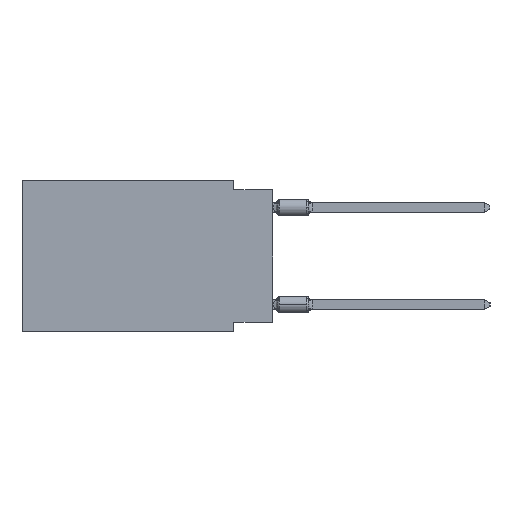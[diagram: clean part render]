
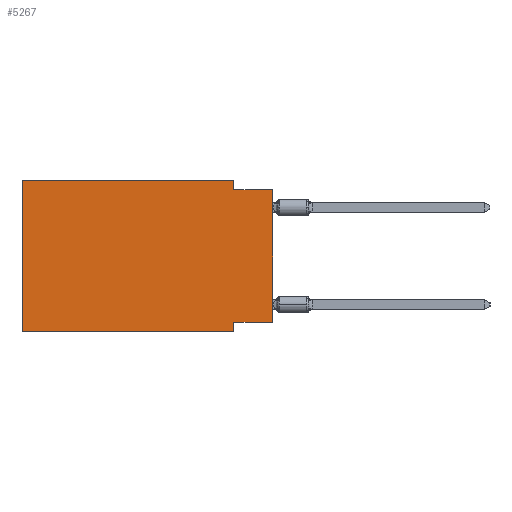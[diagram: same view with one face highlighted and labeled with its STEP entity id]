
A CAD part, left-side view. The second image highlights one B-rep face of the part: STEP entity #5267.
In plain terms, the highlighted planar face has unit normal (-1, 0, 0).
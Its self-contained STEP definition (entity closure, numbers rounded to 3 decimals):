
#580 = EDGE_CURVE ( 'NONE', #13527, #42944, #2707, .T. ) ;
#1333 = CARTESIAN_POINT ( 'NONE',  ( 0., 16.383, -9.906 ) ) ;
#2685 = EDGE_LOOP ( 'NONE', ( #35962, #48918, #42064, #32607, #46112, #20732, #15346, #41713 ) ) ;
#2707 = LINE ( 'NONE', #3240, #50632 ) ;
#3240 = CARTESIAN_POINT ( 'NONE',  ( 0., 2.54, 0. ) ) ;
#3360 = CARTESIAN_POINT ( 'NONE',  ( 0., 0., 0. ) ) ;
#3533 = VERTEX_POINT ( 'NONE', #42495 ) ;
#4226 = CARTESIAN_POINT ( 'NONE',  ( 0., 0., -0.635 ) ) ;
#4782 = CARTESIAN_POINT ( 'NONE',  ( 0., 0., -0.635 ) ) ;
#5267 = ADVANCED_FACE ( 'NONE', ( #26654 ), #30990, .F. ) ;
#6909 = EDGE_CURVE ( 'NONE', #37134, #31573, #53526, .T. ) ;
#7393 = LINE ( 'NONE', #15548, #31809 ) ;
#7659 = EDGE_CURVE ( 'NONE', #42944, #31573, #49798, .T. ) ;
#10741 = CARTESIAN_POINT ( 'NONE',  ( 0., 2.54, 0. ) ) ;
#11814 = VECTOR ( 'NONE', #44645, 1000. ) ;
#13527 = VERTEX_POINT ( 'NONE', #10741 ) ;
#14663 = LINE ( 'NONE', #19260, #47544 ) ;
#14776 = VERTEX_POINT ( 'NONE', #1333 ) ;
#15346 = ORIENTED_EDGE ( 'NONE', *, *, #29718, .F. ) ;
#15548 = CARTESIAN_POINT ( 'NONE',  ( 0., 0., -9.271 ) ) ;
#16994 = DIRECTION ( 'NONE',  ( 0., -1., 0. ) ) ;
#19260 = CARTESIAN_POINT ( 'NONE',  ( 0., 2.54, -9.906 ) ) ;
#20732 = ORIENTED_EDGE ( 'NONE', *, *, #52183, .T. ) ;
#21675 = CARTESIAN_POINT ( 'NONE',  ( 0., 16.383, 0. ) ) ;
#23773 = LINE ( 'NONE', #40573, #53004 ) ;
#26654 = FACE_OUTER_BOUND ( 'NONE', #2685, .T. ) ;
#27711 = EDGE_CURVE ( 'NONE', #37134, #48966, #7393, .T. ) ;
#28843 = VECTOR ( 'NONE', #33619, 1000. ) ;
#29718 = EDGE_CURVE ( 'NONE', #48966, #42482, #14663, .T. ) ;
#29773 = CARTESIAN_POINT ( 'NONE',  ( 0., 2.54, -9.906 ) ) ;
#30990 = PLANE ( 'NONE',  #34425 ) ;
#31573 = VERTEX_POINT ( 'NONE', #4782 ) ;
#31809 = VECTOR ( 'NONE', #32103, 1000. ) ;
#32103 = DIRECTION ( 'NONE',  ( 0., 1., 0. ) ) ;
#32607 = ORIENTED_EDGE ( 'NONE', *, *, #36961, .F. ) ;
#33527 = DIRECTION ( 'NONE',  ( 1., 0., 0. ) ) ;
#33619 = DIRECTION ( 'NONE',  ( 0., -1., 0. ) ) ;
#34425 = AXIS2_PLACEMENT_3D ( 'NONE', #47516, #33527, #43719 ) ;
#35468 = CARTESIAN_POINT ( 'NONE',  ( 0., 0., -9.271 ) ) ;
#35962 = ORIENTED_EDGE ( 'NONE', *, *, #6909, .T. ) ;
#36961 = EDGE_CURVE ( 'NONE', #3533, #13527, #49593, .T. ) ;
#37134 = VERTEX_POINT ( 'NONE', #35468 ) ;
#37583 = CARTESIAN_POINT ( 'NONE',  ( 0., 2.54, -0.635 ) ) ;
#39864 = DIRECTION ( 'NONE',  ( 0., 0., -1. ) ) ;
#40033 = LINE ( 'NONE', #53312, #11814 ) ;
#40573 = CARTESIAN_POINT ( 'NONE',  ( 0., 16.383, -9.906 ) ) ;
#40942 = DIRECTION ( 'NONE',  ( 0., 0., -1. ) ) ;
#41713 = ORIENTED_EDGE ( 'NONE', *, *, #27711, .F. ) ;
#42064 = ORIENTED_EDGE ( 'NONE', *, *, #580, .F. ) ;
#42241 = CARTESIAN_POINT ( 'NONE',  ( 0., 2.54, -9.271 ) ) ;
#42482 = VERTEX_POINT ( 'NONE', #29773 ) ;
#42495 = CARTESIAN_POINT ( 'NONE',  ( 0., 16.383, 0. ) ) ;
#42944 = VERTEX_POINT ( 'NONE', #37583 ) ;
#43719 = DIRECTION ( 'NONE',  ( 0., 0., -1. ) ) ;
#44129 = EDGE_CURVE ( 'NONE', #14776, #3533, #40033, .T. ) ;
#44645 = DIRECTION ( 'NONE',  ( 0., 0., 1. ) ) ;
#45828 = VECTOR ( 'NONE', #16994, 1000. ) ;
#46112 = ORIENTED_EDGE ( 'NONE', *, *, #44129, .F. ) ;
#47516 = CARTESIAN_POINT ( 'NONE',  ( 0., 16.383, 0. ) ) ;
#47544 = VECTOR ( 'NONE', #39864, 1000. ) ;
#47904 = DIRECTION ( 'NONE',  ( 0., -1., 0. ) ) ;
#48918 = ORIENTED_EDGE ( 'NONE', *, *, #7659, .F. ) ;
#48966 = VERTEX_POINT ( 'NONE', #42241 ) ;
#49194 = DIRECTION ( 'NONE',  ( 0., 0., 1. ) ) ;
#49593 = LINE ( 'NONE', #21675, #28843 ) ;
#49798 = LINE ( 'NONE', #4226, #45828 ) ;
#50632 = VECTOR ( 'NONE', #40942, 1000. ) ;
#51854 = VECTOR ( 'NONE', #49194, 1000. ) ;
#52183 = EDGE_CURVE ( 'NONE', #14776, #42482, #23773, .T. ) ;
#53004 = VECTOR ( 'NONE', #47904, 1000. ) ;
#53312 = CARTESIAN_POINT ( 'NONE',  ( 0., 16.383, 0. ) ) ;
#53526 = LINE ( 'NONE', #3360, #51854 ) ;
